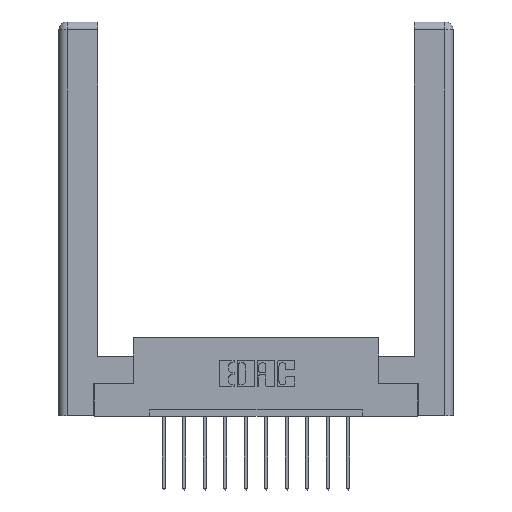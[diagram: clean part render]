
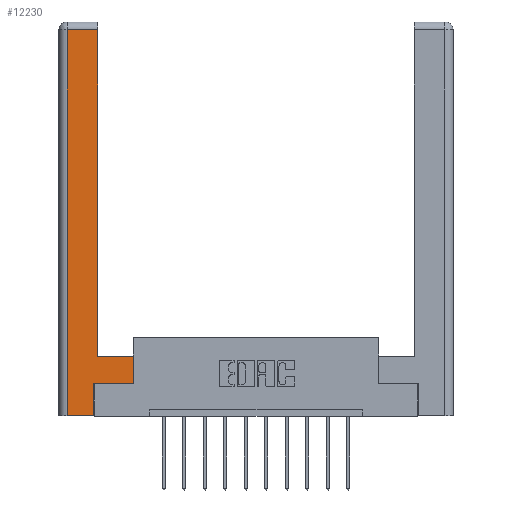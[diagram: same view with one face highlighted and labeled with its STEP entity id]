
A CAD part, top view. The second image highlights one B-rep face of the part: STEP entity #12230.
In plain terms, the highlighted planar face has unit normal (0, 0, 1).
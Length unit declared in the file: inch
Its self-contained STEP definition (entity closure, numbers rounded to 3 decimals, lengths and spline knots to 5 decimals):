
#89 = VECTOR ( 'NONE', #10554, 39.37008 ) ;
#269 = CARTESIAN_POINT ( 'NONE',  ( 0.295, 2.94, 0. ) ) ;
#403 = DIRECTION ( 'NONE',  ( -1., 0., 0. ) ) ;
#522 = CARTESIAN_POINT ( 'NONE',  ( 0.565, 0.45, 0. ) ) ;
#637 = EDGE_LOOP ( 'NONE', ( #5580, #4312, #1652, #4560, #4863, #2321, #10522, #11856 ) ) ;
#808 = EDGE_CURVE ( 'NONE', #12582, #11152, #1925, .T. ) ;
#1392 = EDGE_CURVE ( 'NONE', #7513, #12582, #7770, .T. ) ;
#1413 = CARTESIAN_POINT ( 'NONE',  ( 0.265, 0., 0. ) ) ;
#1556 = VERTEX_POINT ( 'NONE', #13609 ) ;
#1608 = DIRECTION ( 'NONE',  ( 0., -1., 0. ) ) ;
#1652 = ORIENTED_EDGE ( 'NONE', *, *, #1392, .T. ) ;
#1925 = LINE ( 'NONE', #8490, #2594 ) ;
#2143 = PLANE ( 'NONE',  #10061 ) ;
#2251 = EDGE_CURVE ( 'NONE', #7528, #10226, #11134, .T. ) ;
#2321 = ORIENTED_EDGE ( 'NONE', *, *, #2251, .T. ) ;
#2594 = VECTOR ( 'NONE', #11763, 39.37008 ) ;
#2718 = EDGE_CURVE ( 'NONE', #11521, #1556, #7017, .T. ) ;
#2778 = CARTESIAN_POINT ( 'NONE',  ( 0.265, 0.245, 0. ) ) ;
#3643 = VECTOR ( 'NONE', #3887, 39.37008 ) ;
#3666 = LINE ( 'NONE', #10704, #8142 ) ;
#3887 = DIRECTION ( 'NONE',  ( 0., 1., 0. ) ) ;
#4153 = DIRECTION ( 'NONE',  ( 0., 1., 0. ) ) ;
#4312 = ORIENTED_EDGE ( 'NONE', *, *, #9928, .T. ) ;
#4361 = DIRECTION ( 'NONE',  ( 0., 0., -1. ) ) ;
#4560 = ORIENTED_EDGE ( 'NONE', *, *, #808, .T. ) ;
#4863 = ORIENTED_EDGE ( 'NONE', *, *, #11663, .T. ) ;
#5062 = CARTESIAN_POINT ( 'NONE',  ( 0.0615, 2.94, 0. ) ) ;
#5298 = LINE ( 'NONE', #8568, #14219 ) ;
#5332 = VECTOR ( 'NONE', #10926, 39.37008 ) ;
#5459 = DIRECTION ( 'NONE',  ( -1., 0., 0. ) ) ;
#5580 = ORIENTED_EDGE ( 'NONE', *, *, #10750, .T. ) ;
#5787 = LINE ( 'NONE', #5062, #89 ) ;
#6658 = CARTESIAN_POINT ( 'NONE',  ( 0.0615, 2.94, 0. ) ) ;
#6679 = CARTESIAN_POINT ( 'NONE',  ( 0.0615, 0., 0. ) ) ;
#7017 = LINE ( 'NONE', #10328, #14246 ) ;
#7513 = VERTEX_POINT ( 'NONE', #6658 ) ;
#7528 = VERTEX_POINT ( 'NONE', #13075 ) ;
#7770 = LINE ( 'NONE', #12507, #13078 ) ;
#8142 = VECTOR ( 'NONE', #4153, 39.37008 ) ;
#8490 = CARTESIAN_POINT ( 'NONE',  ( 0.265, 0., 0. ) ) ;
#8568 = CARTESIAN_POINT ( 'NONE',  ( 0.565, 0.45, 0. ) ) ;
#8730 = CARTESIAN_POINT ( 'NONE',  ( 0.565, 0.245, 0. ) ) ;
#8959 = EDGE_CURVE ( 'NONE', #10226, #11521, #5298, .T. ) ;
#9706 = CARTESIAN_POINT ( 'NONE',  ( 0., 0., 0. ) ) ;
#9928 = EDGE_CURVE ( 'NONE', #10809, #7513, #5787, .T. ) ;
#10061 = AXIS2_PLACEMENT_3D ( 'NONE', #9706, #4361, #5459 ) ;
#10226 = VERTEX_POINT ( 'NONE', #13860 ) ;
#10328 = CARTESIAN_POINT ( 'NONE',  ( 0.295, 0.45, 0. ) ) ;
#10522 = ORIENTED_EDGE ( 'NONE', *, *, #8959, .T. ) ;
#10554 = DIRECTION ( 'NONE',  ( -1., 0., 0. ) ) ;
#10704 = CARTESIAN_POINT ( 'NONE',  ( 0.295, 3., 0. ) ) ;
#10750 = EDGE_CURVE ( 'NONE', #1556, #10809, #3666, .T. ) ;
#10809 = VERTEX_POINT ( 'NONE', #269 ) ;
#10926 = DIRECTION ( 'NONE',  ( 1., 0., 0. ) ) ;
#11134 = LINE ( 'NONE', #8730, #5332 ) ;
#11152 = VERTEX_POINT ( 'NONE', #1413 ) ;
#11521 = VERTEX_POINT ( 'NONE', #522 ) ;
#11663 = EDGE_CURVE ( 'NONE', #11152, #7528, #14142, .T. ) ;
#11763 = DIRECTION ( 'NONE',  ( 1., 0., 0. ) ) ;
#11856 = ORIENTED_EDGE ( 'NONE', *, *, #2718, .T. ) ;
#12230 = ADVANCED_FACE ( 'NONE', ( #13583 ), #2143, .F. ) ;
#12507 = CARTESIAN_POINT ( 'NONE',  ( 0.0615, 0., 0. ) ) ;
#12582 = VERTEX_POINT ( 'NONE', #6679 ) ;
#13017 = DIRECTION ( 'NONE',  ( 0., 1., 0. ) ) ;
#13075 = CARTESIAN_POINT ( 'NONE',  ( 0.265, 0.245, 0. ) ) ;
#13078 = VECTOR ( 'NONE', #1608, 39.37008 ) ;
#13583 = FACE_OUTER_BOUND ( 'NONE', #637, .T. ) ;
#13609 = CARTESIAN_POINT ( 'NONE',  ( 0.295, 0.45, 0. ) ) ;
#13860 = CARTESIAN_POINT ( 'NONE',  ( 0.565, 0.245, 0. ) ) ;
#14142 = LINE ( 'NONE', #2778, #3643 ) ;
#14219 = VECTOR ( 'NONE', #13017, 39.37008 ) ;
#14246 = VECTOR ( 'NONE', #403, 39.37008 ) ;
